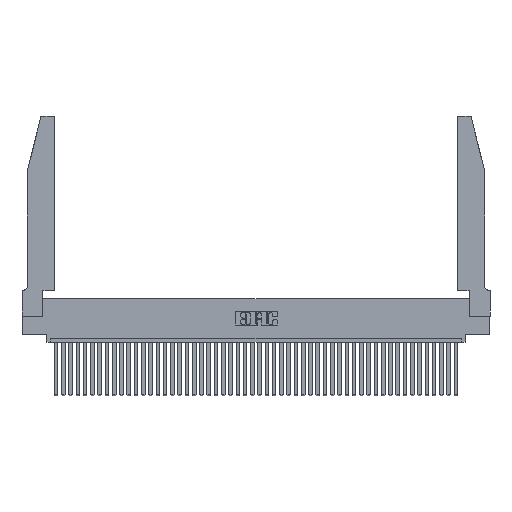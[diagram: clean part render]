
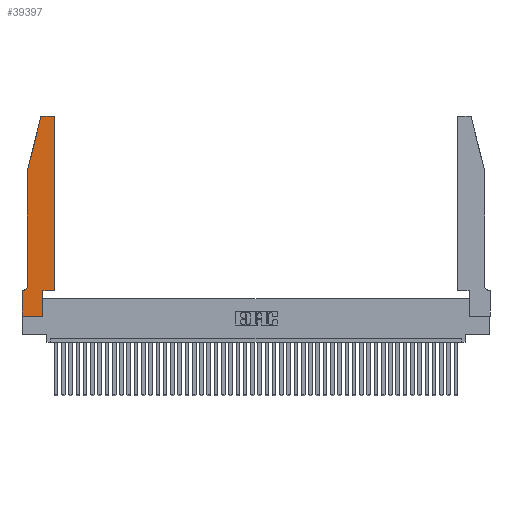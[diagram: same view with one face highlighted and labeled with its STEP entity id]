
A CAD part, top view. The second image highlights one B-rep face of the part: STEP entity #39397.
In plain terms, the highlighted planar face has unit normal (0, 0, 1).
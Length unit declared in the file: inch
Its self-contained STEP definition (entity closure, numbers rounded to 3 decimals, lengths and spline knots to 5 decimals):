
#31 = CARTESIAN_POINT ( 'NONE',  ( 0., 0., 0.37 ) ) ;
#102 = DIRECTION ( 'NONE',  ( 1., 0., 0. ) ) ;
#767 = CARTESIAN_POINT ( 'NONE',  ( 0.2865, 0.35, 0.37 ) ) ;
#796 = ORIENTED_EDGE ( 'NONE', *, *, #37562, .T. ) ;
#813 = ORIENTED_EDGE ( 'NONE', *, *, #1855, .T. ) ;
#1073 = CARTESIAN_POINT ( 'NONE',  ( 0.2865, 0.35, 0.37 ) ) ;
#1257 = VERTEX_POINT ( 'NONE', #9476 ) ;
#1336 = CARTESIAN_POINT ( 'NONE',  ( 0.4505, 0.35, 0.37 ) ) ;
#1401 = EDGE_CURVE ( 'NONE', #13672, #1257, #10541, .T. ) ;
#1582 = DIRECTION ( 'NONE',  ( 1., 0., 0. ) ) ;
#1855 = EDGE_CURVE ( 'NONE', #8902, #4420, #2403, .T. ) ;
#1947 = DIRECTION ( 'NONE',  ( 0., 0., 1. ) ) ;
#2048 = VECTOR ( 'NONE', #11393, 39.37008 ) ;
#2403 = LINE ( 'NONE', #21537, #30123 ) ;
#2695 = DIRECTION ( 'NONE',  ( 0., 0., 1. ) ) ;
#3964 = AXIS2_PLACEMENT_3D ( 'NONE', #44293, #2695, #102 ) ;
#4151 = LINE ( 'NONE', #27040, #36805 ) ;
#4420 = VERTEX_POINT ( 'NONE', #38787 ) ;
#4578 = EDGE_CURVE ( 'NONE', #20900, #8902, #15083, .T. ) ;
#5322 = EDGE_CURVE ( 'NONE', #4420, #44035, #16245, .T. ) ;
#6153 = CARTESIAN_POINT ( 'NONE',  ( 0.284, 2.75, 0.37 ) ) ;
#6556 = DIRECTION ( 'NONE',  ( 0., -1., 0. ) ) ;
#6984 = ORIENTED_EDGE ( 'NONE', *, *, #31361, .T. ) ;
#7688 = DIRECTION ( 'NONE',  ( -0.239, -0.971, 0. ) ) ;
#7725 = DIRECTION ( 'NONE',  ( 0., 1., 0. ) ) ;
#7821 = LINE ( 'NONE', #31, #28502 ) ;
#7863 = AXIS2_PLACEMENT_3D ( 'NONE', #19780, #30735, #34071 ) ;
#8902 = VERTEX_POINT ( 'NONE', #33933 ) ;
#9476 = CARTESIAN_POINT ( 'NONE',  ( 0., 0.35, 0.37 ) ) ;
#9808 = ORIENTED_EDGE ( 'NONE', *, *, #14098, .T. ) ;
#10454 = VERTEX_POINT ( 'NONE', #16983 ) ;
#10541 = LINE ( 'NONE', #19006, #43162 ) ;
#10679 = ORIENTED_EDGE ( 'NONE', *, *, #5322, .T. ) ;
#11238 = CARTESIAN_POINT ( 'NONE',  ( 0., 0., 0.37 ) ) ;
#11393 = DIRECTION ( 'NONE',  ( 1., 0., 0. ) ) ;
#11793 = ORIENTED_EDGE ( 'NONE', *, *, #28977, .T. ) ;
#12064 = CARTESIAN_POINT ( 'NONE',  ( 0.4205, 2.75, 0.37 ) ) ;
#12083 = CARTESIAN_POINT ( 'NONE',  ( 0.4205, 2.72, 0.37 ) ) ;
#13307 = VERTEX_POINT ( 'NONE', #12064 ) ;
#13672 = VERTEX_POINT ( 'NONE', #27205 ) ;
#13920 = LINE ( 'NONE', #28930, #2048 ) ;
#14098 = EDGE_CURVE ( 'NONE', #10454, #13307, #44274, .T. ) ;
#14649 = CARTESIAN_POINT ( 'NONE',  ( 0.4505, 0.35, 0.37 ) ) ;
#15071 = VERTEX_POINT ( 'NONE', #30443 ) ;
#15083 = CIRCLE ( 'NONE', #3964, 0.03 ) ;
#15273 = ORIENTED_EDGE ( 'NONE', *, *, #4578, .T. ) ;
#15556 = DIRECTION ( 'NONE',  ( 1., 0., 0. ) ) ;
#16030 = AXIS2_PLACEMENT_3D ( 'NONE', #36370, #25403, #1582 ) ;
#16245 = LINE ( 'NONE', #44980, #19982 ) ;
#16983 = CARTESIAN_POINT ( 'NONE',  ( 0.4505, 2.72, 0.37 ) ) ;
#17352 = VERTEX_POINT ( 'NONE', #1336 ) ;
#18513 = FACE_OUTER_BOUND ( 'NONE', #20807, .T. ) ;
#18647 = ORIENTED_EDGE ( 'NONE', *, *, #23045, .T. ) ;
#19006 = CARTESIAN_POINT ( 'NONE',  ( 0.0755, 0.35, 0.37 ) ) ;
#19726 = CARTESIAN_POINT ( 'NONE',  ( 0., 0., 0.37 ) ) ;
#19780 = CARTESIAN_POINT ( 'NONE',  ( 0.0055, 0.42, 0.37 ) ) ;
#19982 = VECTOR ( 'NONE', #6556, 39.37008 ) ;
#20807 = EDGE_LOOP ( 'NONE', ( #22132, #15273, #813, #10679, #11793, #35933, #6984, #44067, #27373, #796, #18647, #9808 ) ) ;
#20900 = VERTEX_POINT ( 'NONE', #6153 ) ;
#21537 = CARTESIAN_POINT ( 'NONE',  ( 0.0755, 2., 0.37 ) ) ;
#22132 = ORIENTED_EDGE ( 'NONE', *, *, #25373, .T. ) ;
#22719 = EDGE_CURVE ( 'NONE', #15071, #25768, #29944, .T. ) ;
#23045 = EDGE_CURVE ( 'NONE', #17352, #10454, #39694, .T. ) ;
#23637 = VECTOR ( 'NONE', #43719, 39.37008 ) ;
#23833 = DIRECTION ( 'NONE',  ( -1., 0., 0. ) ) ;
#25373 = EDGE_CURVE ( 'NONE', #13307, #20900, #4151, .T. ) ;
#25403 = DIRECTION ( 'NONE',  ( 0., 0., 1. ) ) ;
#25768 = VERTEX_POINT ( 'NONE', #1073 ) ;
#27040 = CARTESIAN_POINT ( 'NONE',  ( 0.2605, 2.75, 0.37 ) ) ;
#27205 = CARTESIAN_POINT ( 'NONE',  ( 0.0055, 0.35, 0.37 ) ) ;
#27373 = ORIENTED_EDGE ( 'NONE', *, *, #22719, .T. ) ;
#27918 = VERTEX_POINT ( 'NONE', #11238 ) ;
#28502 = VECTOR ( 'NONE', #40057, 39.37008 ) ;
#28930 = CARTESIAN_POINT ( 'NONE',  ( 0.4505, 0.35, 0.37 ) ) ;
#28977 = EDGE_CURVE ( 'NONE', #44035, #13672, #37374, .T. ) ;
#29412 = VECTOR ( 'NONE', #7725, 39.37008 ) ;
#29944 = LINE ( 'NONE', #767, #29412 ) ;
#30123 = VECTOR ( 'NONE', #7688, 39.37008 ) ;
#30443 = CARTESIAN_POINT ( 'NONE',  ( 0.2865, 0., 0.37 ) ) ;
#30735 = DIRECTION ( 'NONE',  ( 0., 0., -1. ) ) ;
#31361 = EDGE_CURVE ( 'NONE', #1257, #27918, #7821, .T. ) ;
#32840 = DIRECTION ( 'NONE',  ( -1., 0., 0. ) ) ;
#33933 = CARTESIAN_POINT ( 'NONE',  ( 0.25487, 2.72718, 0.37 ) ) ;
#34071 = DIRECTION ( 'NONE',  ( -1., 0., 0. ) ) ;
#34805 = VECTOR ( 'NONE', #42051, 39.37008 ) ;
#35022 = LINE ( 'NONE', #19726, #23637 ) ;
#35933 = ORIENTED_EDGE ( 'NONE', *, *, #1401, .T. ) ;
#36370 = CARTESIAN_POINT ( 'NONE',  ( 0., 0.35, 0.37 ) ) ;
#36406 = AXIS2_PLACEMENT_3D ( 'NONE', #12083, #1947, #15556 ) ;
#36805 = VECTOR ( 'NONE', #23833, 39.37008 ) ;
#37374 = CIRCLE ( 'NONE', #7863, 0.07 ) ;
#37562 = EDGE_CURVE ( 'NONE', #25768, #17352, #13920, .T. ) ;
#38586 = CARTESIAN_POINT ( 'NONE',  ( 0.0755, 0.42, 0.37 ) ) ;
#38787 = CARTESIAN_POINT ( 'NONE',  ( 0.0755, 2., 0.37 ) ) ;
#39397 = ADVANCED_FACE ( 'NONE', ( #18513 ), #39549, .T. ) ;
#39549 = PLANE ( 'NONE',  #16030 ) ;
#39694 = LINE ( 'NONE', #14649, #34805 ) ;
#40057 = DIRECTION ( 'NONE',  ( 0., -1., 0. ) ) ;
#42051 = DIRECTION ( 'NONE',  ( 0., 1., 0. ) ) ;
#42744 = EDGE_CURVE ( 'NONE', #27918, #15071, #35022, .T. ) ;
#43162 = VECTOR ( 'NONE', #32840, 39.37008 ) ;
#43719 = DIRECTION ( 'NONE',  ( 1., 0., 0. ) ) ;
#44035 = VERTEX_POINT ( 'NONE', #38586 ) ;
#44067 = ORIENTED_EDGE ( 'NONE', *, *, #42744, .T. ) ;
#44274 = CIRCLE ( 'NONE', #36406, 0.03 ) ;
#44293 = CARTESIAN_POINT ( 'NONE',  ( 0.284, 2.72, 0.37 ) ) ;
#44980 = CARTESIAN_POINT ( 'NONE',  ( 0.0755, 2., 0.37 ) ) ;
